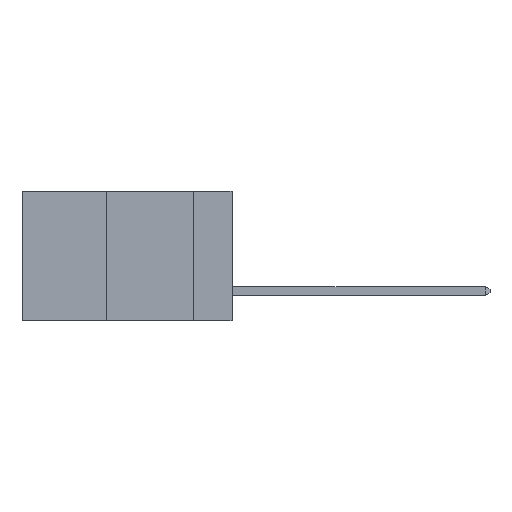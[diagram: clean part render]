
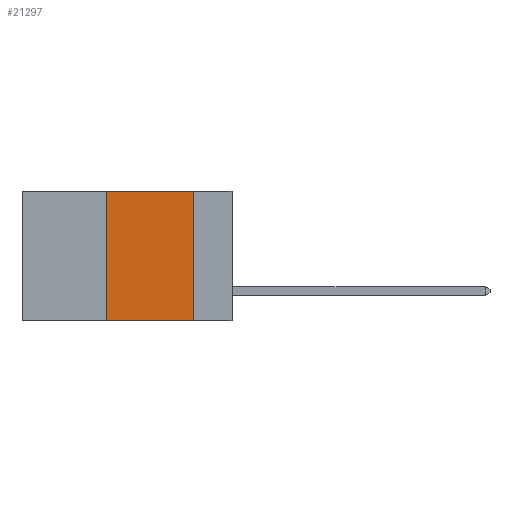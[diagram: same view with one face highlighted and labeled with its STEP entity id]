
A CAD part, left-side view. The second image highlights one B-rep face of the part: STEP entity #21297.
In plain terms, the highlighted planar face has unit normal (-1, 0, 0).
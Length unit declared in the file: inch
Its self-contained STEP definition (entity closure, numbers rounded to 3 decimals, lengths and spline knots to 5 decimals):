
#224 = CARTESIAN_POINT ( 'NONE',  ( 0., 0.6, 0. ) ) ;
#581 = DIRECTION ( 'NONE',  ( 0., 0., -1. ) ) ;
#762 = CARTESIAN_POINT ( 'NONE',  ( 0., 0.36, -0.37 ) ) ;
#1110 = EDGE_LOOP ( 'NONE', ( #20096, #21219, #3832, #15016 ) ) ;
#1571 = LINE ( 'NONE', #224, #20360 ) ;
#1939 = CARTESIAN_POINT ( 'NONE',  ( 0., 0.6, -0.37 ) ) ;
#3291 = CARTESIAN_POINT ( 'NONE',  ( 0., 0.11, 0. ) ) ;
#3832 = ORIENTED_EDGE ( 'NONE', *, *, #12897, .F. ) ;
#5797 = VERTEX_POINT ( 'NONE', #19639 ) ;
#6588 = EDGE_CURVE ( 'NONE', #15728, #5797, #19353, .T. ) ;
#7101 = VECTOR ( 'NONE', #23963, 39.37008 ) ;
#9857 = FACE_OUTER_BOUND ( 'NONE', #1110, .T. ) ;
#11919 = DIRECTION ( 'NONE',  ( 1., 0., 0. ) ) ;
#12579 = AXIS2_PLACEMENT_3D ( 'NONE', #22915, #11919, #581 ) ;
#12667 = CARTESIAN_POINT ( 'NONE',  ( 0., 0.36, 0. ) ) ;
#12897 = EDGE_CURVE ( 'NONE', #15728, #23416, #16552, .T. ) ;
#13017 = CARTESIAN_POINT ( 'NONE',  ( 0., 0.36, 0. ) ) ;
#15016 = ORIENTED_EDGE ( 'NONE', *, *, #6588, .T. ) ;
#15462 = DIRECTION ( 'NONE',  ( 0., -1., 0. ) ) ;
#15728 = VERTEX_POINT ( 'NONE', #762 ) ;
#16552 = LINE ( 'NONE', #13017, #7101 ) ;
#18352 = LINE ( 'NONE', #3291, #23667 ) ;
#19353 = LINE ( 'NONE', #1939, #22945 ) ;
#19370 = CARTESIAN_POINT ( 'NONE',  ( 0., 0.11, 0. ) ) ;
#19639 = CARTESIAN_POINT ( 'NONE',  ( 0., 0.11, -0.37 ) ) ;
#20096 = ORIENTED_EDGE ( 'NONE', *, *, #21580, .F. ) ;
#20360 = VECTOR ( 'NONE', #15462, 39.37008 ) ;
#21160 = PLANE ( 'NONE',  #12579 ) ;
#21219 = ORIENTED_EDGE ( 'NONE', *, *, #22598, .F. ) ;
#21297 = ADVANCED_FACE ( 'NONE', ( #9857 ), #21160, .F. ) ;
#21580 = EDGE_CURVE ( 'NONE', #22653, #5797, #18352, .T. ) ;
#21890 = DIRECTION ( 'NONE',  ( 0., 0., -1. ) ) ;
#22467 = DIRECTION ( 'NONE',  ( 0., -1., 0. ) ) ;
#22598 = EDGE_CURVE ( 'NONE', #23416, #22653, #1571, .T. ) ;
#22653 = VERTEX_POINT ( 'NONE', #19370 ) ;
#22915 = CARTESIAN_POINT ( 'NONE',  ( 0., 0.6, 0. ) ) ;
#22945 = VECTOR ( 'NONE', #22467, 39.37008 ) ;
#23416 = VERTEX_POINT ( 'NONE', #12667 ) ;
#23667 = VECTOR ( 'NONE', #21890, 39.37008 ) ;
#23963 = DIRECTION ( 'NONE',  ( 0., 0., 1. ) ) ;
